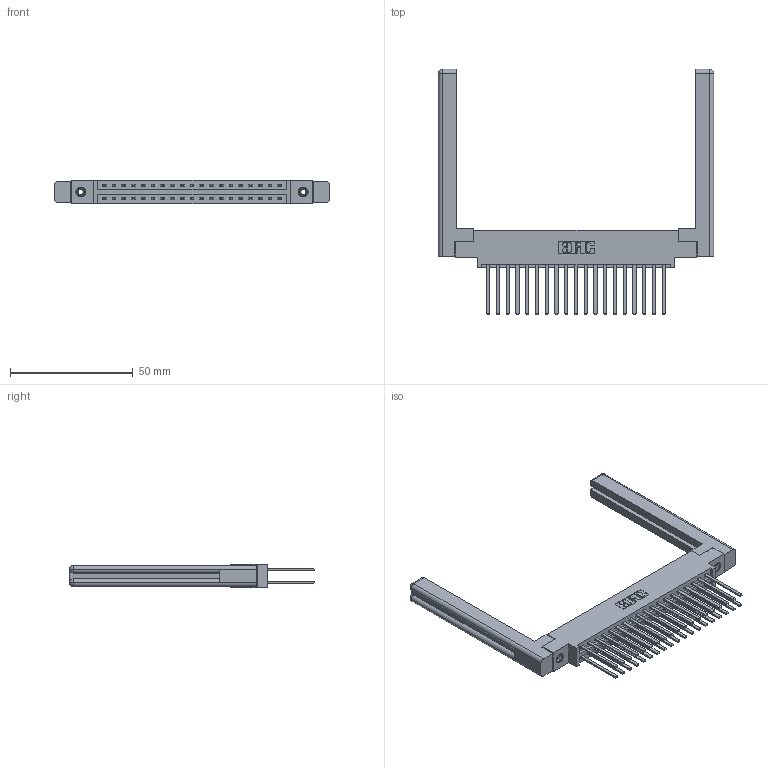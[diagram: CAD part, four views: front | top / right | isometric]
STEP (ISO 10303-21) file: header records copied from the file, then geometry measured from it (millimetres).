
FILE_DESCRIPTION (( 'STEP AP203' ), '1' );
FILE_NAME ('387-038-544-858.STEP', '2019-10-17T21:57:47', ( '' ), ( '' ), 'SwSTEP 2.0', 'SolidWorks 2016', '' );
FILE_SCHEMA (( 'CONFIG_CONTROL_DESIGN' ));
Length unit declared in the file: inch
Products named in the file (5): 345-292-001_345-293-144; 307-220-058; 387-038-544-858; 345-250-001_345-250-001-102; 337 Part_0.170 Offset - 0.156 Dia-TI
Assembly tree (43 placements, depth 2):
  387-038-544-858
    337 Part_0.170 Offset - 0.156 Dia-TI
    345-292-001_345-293-144  x38
    345-250-001_345-250-001-102  x2
    307-220-058  x2
Bounding box: 111.91 x 99.7 x 9.4 mm (x, y, z)
Volume: 19045.6 mm3; surface area: 20128 mm2
Topology: 43 solids, 43 shells, 2084 faces, 6111 edges, 4010 vertices
Faces by surface type: plane 1450, cylinder 610, cone 12, torus 12
Entity records: 20288 total; most frequent: CARTESIAN_POINT 3445, ORIENTED_EDGE 3320, DIRECTION 2984, EDGE_CURVE 1660, LINE 1488, VECTOR 1488, VERTEX_POINT 1098, AXIS2_PLACEMENT_3D 748
